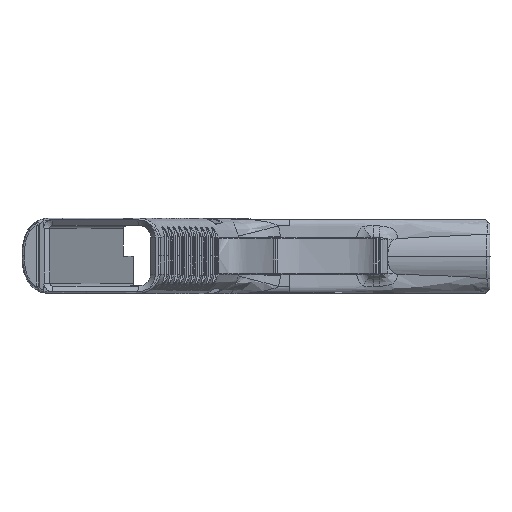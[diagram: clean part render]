
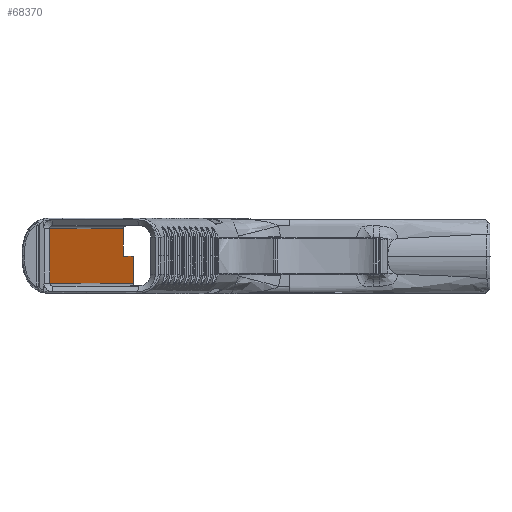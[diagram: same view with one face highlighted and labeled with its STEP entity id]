
A CAD part, top view. The second image highlights one B-rep face of the part: STEP entity #68370.
In plain terms, the highlighted planar face has unit normal (0.951, 0, 0.309).
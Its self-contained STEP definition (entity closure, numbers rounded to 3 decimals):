
#517 = VERTEX_POINT ( 'NONE', #129990 ) ;
#1186 = ORIENTED_EDGE ( 'NONE', *, *, #61879, .F. ) ;
#4240 = LINE ( 'NONE', #245933, #99634 ) ;
#11002 = DIRECTION ( 'NONE',  ( -0.309, 0., 0.951 ) ) ;
#28046 = VERTEX_POINT ( 'NONE', #45852 ) ;
#30025 = EDGE_CURVE ( 'NONE', #517, #28046, #95564, .T. ) ;
#35303 = LINE ( 'NONE', #254101, #159076 ) ;
#45852 = CARTESIAN_POINT ( 'NONE',  ( 49.444, 9.399, -88.458 ) ) ;
#57054 = PLANE ( 'NONE',  #149013 ) ;
#60803 = ORIENTED_EDGE ( 'NONE', *, *, #30025, .F. ) ;
#60861 = VERTEX_POINT ( 'NONE', #225823 ) ;
#61879 = EDGE_CURVE ( 'NONE', #254306, #60861, #4240, .T. ) ;
#68370 = ADVANCED_FACE ( 'NONE', ( #161912 ), #57054, .F. ) ;
#69357 = CARTESIAN_POINT ( 'NONE',  ( 49.444, 0.002, -88.458 ) ) ;
#81832 = VECTOR ( 'NONE', #214340, 1000. ) ;
#95564 = LINE ( 'NONE', #186088, #140103 ) ;
#99634 = VECTOR ( 'NONE', #103269, 1000. ) ;
#101322 = EDGE_LOOP ( 'NONE', ( #222441, #60803, #186493, #251954, #1186, #138570 ) ) ;
#103269 = DIRECTION ( 'NONE',  ( 0., -1., 0. ) ) ;
#107584 = CARTESIAN_POINT ( 'NONE',  ( 52.695, 0.002, -98.462 ) ) ;
#116990 = VERTEX_POINT ( 'NONE', #146386 ) ;
#121080 = CARTESIAN_POINT ( 'NONE',  ( 52.856, 0.002, -98.958 ) ) ;
#121954 = EDGE_CURVE ( 'NONE', #60861, #116990, #35303, .T. ) ;
#123716 = VERTEX_POINT ( 'NONE', #69357 ) ;
#124366 = EDGE_CURVE ( 'NONE', #123716, #254306, #243764, .T. ) ;
#129990 = CARTESIAN_POINT ( 'NONE',  ( 24.128, 9.399, -10.543 ) ) ;
#135852 = LINE ( 'NONE', #193946, #81832 ) ;
#138570 = ORIENTED_EDGE ( 'NONE', *, *, #124366, .F. ) ;
#140103 = VECTOR ( 'NONE', #165722, 1000. ) ;
#146386 = CARTESIAN_POINT ( 'NONE',  ( 24.128, -9.399, -10.543 ) ) ;
#148415 = DIRECTION ( 'NONE',  ( 0.309, 0., -0.951 ) ) ;
#149013 = AXIS2_PLACEMENT_3D ( 'NONE', #258428, #199018, #219363 ) ;
#159076 = VECTOR ( 'NONE', #11002, 1000. ) ;
#159803 = VECTOR ( 'NONE', #199397, 1000. ) ;
#161912 = FACE_OUTER_BOUND ( 'NONE', #101322, .T. ) ;
#165722 = DIRECTION ( 'NONE',  ( 0.309, 0., -0.951 ) ) ;
#180438 = VECTOR ( 'NONE', #148415, 1000. ) ;
#186088 = CARTESIAN_POINT ( 'NONE',  ( 52.695, 9.399, -98.462 ) ) ;
#186493 = ORIENTED_EDGE ( 'NONE', *, *, #241948, .F. ) ;
#193946 = CARTESIAN_POINT ( 'NONE',  ( 49.444, 0., -88.458 ) ) ;
#199018 = DIRECTION ( 'NONE',  ( -0.951, 0., -0.309 ) ) ;
#199397 = DIRECTION ( 'NONE',  ( 0., 1., 0. ) ) ;
#214340 = DIRECTION ( 'NONE',  ( 0., -1., 0. ) ) ;
#216760 = LINE ( 'NONE', #261453, #159803 ) ;
#219363 = DIRECTION ( 'NONE',  ( -0.309, 0., 0.951 ) ) ;
#222441 = ORIENTED_EDGE ( 'NONE', *, *, #234535, .F. ) ;
#225823 = CARTESIAN_POINT ( 'NONE',  ( 52.856, -9.399, -98.958 ) ) ;
#234535 = EDGE_CURVE ( 'NONE', #28046, #123716, #135852, .T. ) ;
#241948 = EDGE_CURVE ( 'NONE', #116990, #517, #216760, .T. ) ;
#243764 = LINE ( 'NONE', #107584, #180438 ) ;
#245933 = CARTESIAN_POINT ( 'NONE',  ( 52.856, 0.001, -98.958 ) ) ;
#251954 = ORIENTED_EDGE ( 'NONE', *, *, #121954, .F. ) ;
#254101 = CARTESIAN_POINT ( 'NONE',  ( 52.695, -9.399, -98.462 ) ) ;
#254306 = VERTEX_POINT ( 'NONE', #121080 ) ;
#258428 = CARTESIAN_POINT ( 'NONE',  ( 52.695, 0., -98.462 ) ) ;
#261453 = CARTESIAN_POINT ( 'NONE',  ( 24.128, 0., -10.543 ) ) ;
